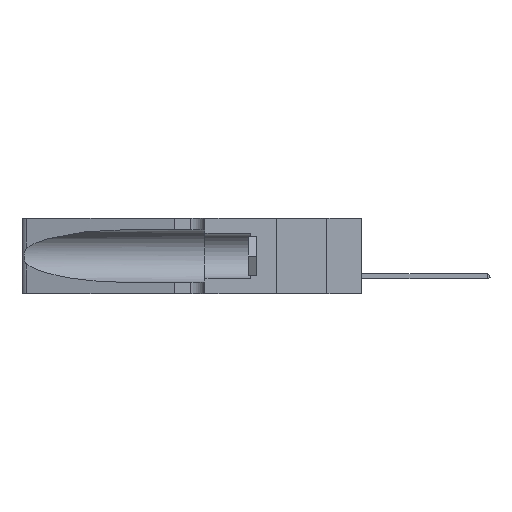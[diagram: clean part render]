
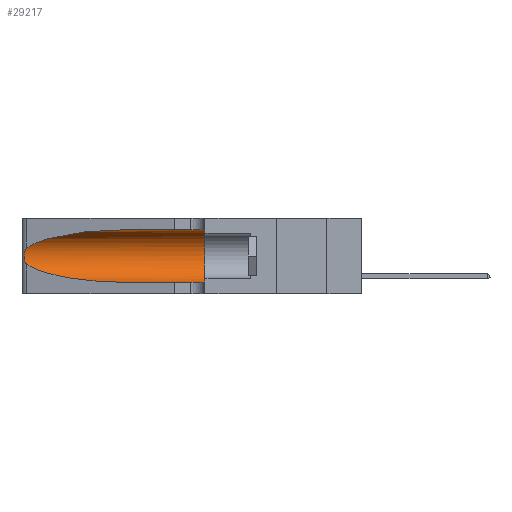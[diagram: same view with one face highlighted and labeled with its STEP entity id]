
A CAD part, left-side view. The second image highlights one B-rep face of the part: STEP entity #29217.
In plain terms, the highlighted cylindrical face has radius 3.308 mm (diameter 6.617 mm), a partial arc.
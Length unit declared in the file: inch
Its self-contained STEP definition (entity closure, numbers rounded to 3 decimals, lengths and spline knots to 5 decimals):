
#442 = CARTESIAN_POINT ( 'NONE',  ( 0.1305, 1.61858, 0.05475 ) ) ;
#790 = EDGE_CURVE ( 'NONE', #15447, #27784, #21722, .T. ) ;
#1030 = VECTOR ( 'NONE', #6055, 39.37008 ) ;
#1583 = CARTESIAN_POINT ( 'NONE',  ( 0.25787, 1.23484, 0.2124 ) ) ;
#1932 = CARTESIAN_POINT ( 'NONE',  ( 0.25487, 1.22718, 0.14631 ) ) ;
#2058 = CARTESIAN_POINT ( 'NONE',  ( 0.2373, 1.15595, 0.28018 ) ) ;
#3053 = VERTEX_POINT ( 'NONE', #32031 ) ;
#4071 = CARTESIAN_POINT ( 'NONE',  ( 0.1305, 0.35, 0.05475 ) ) ;
#4278 = CARTESIAN_POINT ( 'NONE',  ( 0.25854, 1.2359, 0.20912 ) ) ;
#4359 = ORIENTED_EDGE ( 'NONE', *, *, #26864, .T. ) ;
#4523 = VECTOR ( 'NONE', #12266, 39.37008 ) ;
#5701 = DIRECTION ( 'NONE',  ( 0., 0., 1. ) ) ;
#6055 = DIRECTION ( 'NONE',  ( 0., -1., 0. ) ) ;
#6601 = CYLINDRICAL_SURFACE ( 'NONE', #13251, 0.13025 ) ;
#7178 = CARTESIAN_POINT ( 'NONE',  ( 0.26075, 1.23896, 0.178 ) ) ;
#7251 = ORIENTED_EDGE ( 'NONE', *, *, #14614, .T. ) ;
#7289 = CARTESIAN_POINT ( 'NONE',  ( 0.18966, 0.96281, 0.05475 ) ) ;
#8133 = LINE ( 'NONE', #442, #1030 ) ;
#8276 = FACE_OUTER_BOUND ( 'NONE', #24189, .T. ) ;
#9008 = ORIENTED_EDGE ( 'NONE', *, *, #790, .T. ) ;
#9354 = CARTESIAN_POINT ( 'NONE',  ( 0.1305, 0.72297, 0.05475 ) ) ;
#9869 = CARTESIAN_POINT ( 'NONE',  ( 0.25789, 1.23486, 0.15765 ) ) ;
#9876 = CARTESIAN_POINT ( 'NONE',  ( 0.2373, 1.15595, 0.08982 ) ) ;
#11058 = EDGE_CURVE ( 'NONE', #3053, #34553, #24528, .T. ) ;
#11227 = ORIENTED_EDGE ( 'NONE', *, *, #22132, .T. ) ;
#12266 = DIRECTION ( 'NONE',  ( 0., -1., 0. ) ) ;
#12460 = CARTESIAN_POINT ( 'NONE',  ( 0.26075, 1.23896, 0.19203 ) ) ;
#12704 = DIRECTION ( 'NONE',  ( 0., 0., -1. ) ) ;
#12812 = CARTESIAN_POINT ( 'NONE',  ( 0.25487, 1.22718, 0.22369 ) ) ;
#13251 = AXIS2_PLACEMENT_3D ( 'NONE', #28788, #20768, #12704 ) ;
#13352 = ORIENTED_EDGE ( 'NONE', *, *, #11058, .F. ) ;
#13590 = DIRECTION ( 'NONE',  ( 0., 1., 0. ) ) ;
#13722 = CARTESIAN_POINT ( 'NONE',  ( 0.25487, 1.22718, 0.22369 ) ) ;
#14614 = EDGE_CURVE ( 'NONE', #27784, #16189, #8133, .T. ) ;
#14821 = ORIENTED_EDGE ( 'NONE', *, *, #19670, .F. ) ;
#15139 =( BOUNDED_CURVE ( )  B_SPLINE_CURVE ( 3, ( #34075, #34427, #2058, #12812 ),
 .UNSPECIFIED., .F., .T. ) 
 B_SPLINE_CURVE_WITH_KNOTS ( ( 4, 4 ),
 ( 1.5708, 2.84003 ),
 .UNSPECIFIED. ) 
 CURVE ( )  GEOMETRIC_REPRESENTATION_ITEM ( )  RATIONAL_B_SPLINE_CURVE ( ( 1., 0.87, 0.87, 1. ) ) 
 REPRESENTATION_ITEM ( '' )  );
#15284 = CARTESIAN_POINT ( 'NONE',  ( 0.25487, 1.22718, 0.22369 ) ) ;
#15447 = VERTEX_POINT ( 'NONE', #32644 ) ;
#15839 = CIRCLE ( 'NONE', #22978, 0.13025 ) ;
#16189 = VERTEX_POINT ( 'NONE', #4071 ) ;
#17452 = CARTESIAN_POINT ( 'NONE',  ( 0.25639, 1.23184, 0.21858 ) ) ;
#17654 = B_SPLINE_CURVE_WITH_KNOTS ( 'NONE', 3,
 ( #15284, #25767, #17452, #1583, #4278, #25877, #12460, #7178, #28297, #33633, #9869, #17916, #23326, #1932 ),
 .UNSPECIFIED., .F., .F.,
 ( 4, 2, 2, 2, 2, 2, 4 ),
 ( 0., 0.00027, 0.00053, 0.00107, 0.0016, 0.00187, 0.00214 ),
 .UNSPECIFIED. ) ;
#17916 = CARTESIAN_POINT ( 'NONE',  ( 0.25639, 1.23186, 0.15144 ) ) ;
#19670 = EDGE_CURVE ( 'NONE', #34553, #16189, #15839, .T. ) ;
#19952 = CARTESIAN_POINT ( 'NONE',  ( 0.1305, 1.61858, 0.31525 ) ) ;
#20768 = DIRECTION ( 'NONE',  ( 0., -1., 0. ) ) ;
#21716 = CARTESIAN_POINT ( 'NONE',  ( 0.1305, 0.35, 0.185 ) ) ;
#21722 =( BOUNDED_CURVE ( )  B_SPLINE_CURVE ( 3, ( #28302, #9876, #7289, #28418 ),
 .UNSPECIFIED., .F., .T. ) 
 B_SPLINE_CURVE_WITH_KNOTS ( ( 4, 4 ),
 ( 3.44316, 4.71239 ),
 .UNSPECIFIED. ) 
 CURVE ( )  GEOMETRIC_REPRESENTATION_ITEM ( )  RATIONAL_B_SPLINE_CURVE ( ( 1., 0.87, 0.87, 1. ) ) 
 REPRESENTATION_ITEM ( '' )  );
#22132 = EDGE_CURVE ( 'NONE', #34286, #15447, #17654, .T. ) ;
#22978 = AXIS2_PLACEMENT_3D ( 'NONE', #21716, #13590, #5701 ) ;
#23326 = CARTESIAN_POINT ( 'NONE',  ( 0.25555, 1.22993, 0.14849 ) ) ;
#24189 = EDGE_LOOP ( 'NONE', ( #4359, #11227, #9008, #7251, #14821, #13352 ) ) ;
#24528 = LINE ( 'NONE', #19952, #4523 ) ;
#25767 = CARTESIAN_POINT ( 'NONE',  ( 0.25555, 1.22994, 0.2215 ) ) ;
#25877 = CARTESIAN_POINT ( 'NONE',  ( 0.26018, 1.23835, 0.19895 ) ) ;
#26864 = EDGE_CURVE ( 'NONE', #3053, #34286, #15139, .T. ) ;
#27784 = VERTEX_POINT ( 'NONE', #9354 ) ;
#28297 = CARTESIAN_POINT ( 'NONE',  ( 0.26017, 1.23833, 0.17102 ) ) ;
#28302 = CARTESIAN_POINT ( 'NONE',  ( 0.25487, 1.22718, 0.14631 ) ) ;
#28418 = CARTESIAN_POINT ( 'NONE',  ( 0.1305, 0.72297, 0.05475 ) ) ;
#28788 = CARTESIAN_POINT ( 'NONE',  ( 0.1305, 1.61858, 0.185 ) ) ;
#29217 = ADVANCED_FACE ( 'NONE', ( #8276 ), #6601, .F. ) ;
#32031 = CARTESIAN_POINT ( 'NONE',  ( 0.1305, 0.72297, 0.31525 ) ) ;
#32644 = CARTESIAN_POINT ( 'NONE',  ( 0.25487, 1.22718, 0.14631 ) ) ;
#33633 = CARTESIAN_POINT ( 'NONE',  ( 0.25856, 1.23593, 0.16098 ) ) ;
#33922 = CARTESIAN_POINT ( 'NONE',  ( 0.1305, 0.35, 0.31525 ) ) ;
#34075 = CARTESIAN_POINT ( 'NONE',  ( 0.1305, 0.72297, 0.31525 ) ) ;
#34286 = VERTEX_POINT ( 'NONE', #13722 ) ;
#34427 = CARTESIAN_POINT ( 'NONE',  ( 0.18966, 0.96281, 0.31525 ) ) ;
#34553 = VERTEX_POINT ( 'NONE', #33922 ) ;
